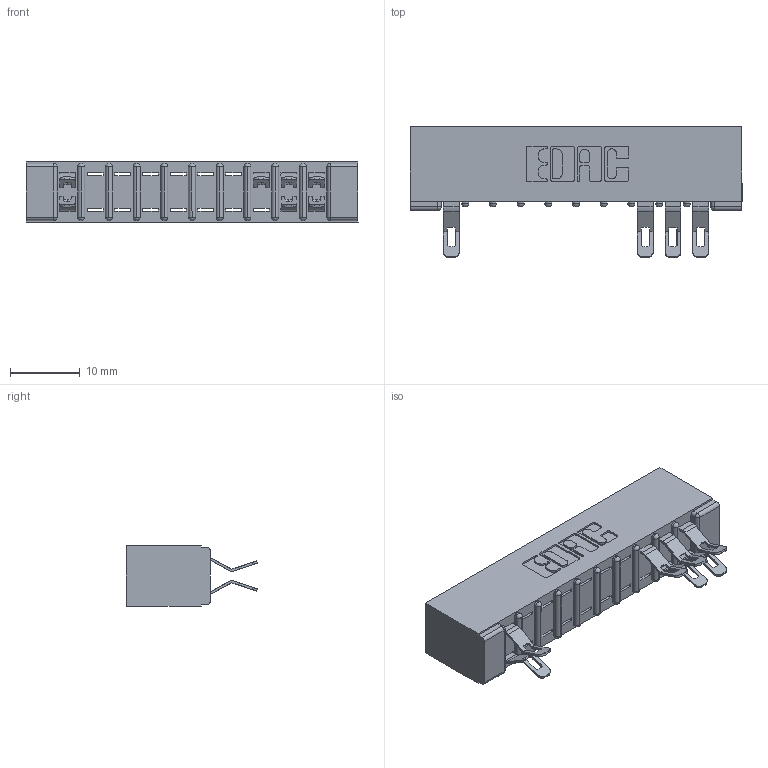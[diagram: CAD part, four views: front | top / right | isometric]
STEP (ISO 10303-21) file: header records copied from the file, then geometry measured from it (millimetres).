
FILE_DESCRIPTION (( 'STEP AP203' ), '1' );
FILE_NAME ('307-020-555-201.STEP', '2018-08-04T01:48:30', ( '' ), ( '' ), 'SwSTEP 2.0', 'SolidWorks 2016', '' );
FILE_SCHEMA (( 'CONFIG_CONTROL_DESIGN' ));
Length unit declared in the file: inch
Products named in the file (3): 307 Part_No Mounting Lugs; 307-290-001_555; 307-020-555-201
Assembly tree (8 placements, depth 2):
  307-020-555-201
    307 Part_No Mounting Lugs
    307-290-001_555  x7
Bounding box: 47.5 x 18.75 x 8.71 mm (x, y, z)
Volume: 3193.9 mm3; surface area: 4607.3 mm2
Topology: 8 solids, 8 shells, 678 faces, 1982 edges, 1280 vertices
Faces by surface type: plane 382, cylinder 274, sphere 22
Entity records: 12681 total; most frequent: CARTESIAN_POINT 2141, ORIENTED_EDGE 2132, DIRECTION 2104, EDGE_CURVE 1066, VECTOR 794, LINE 794, VERTEX_POINT 692, AXIS2_PLACEMENT_3D 655
